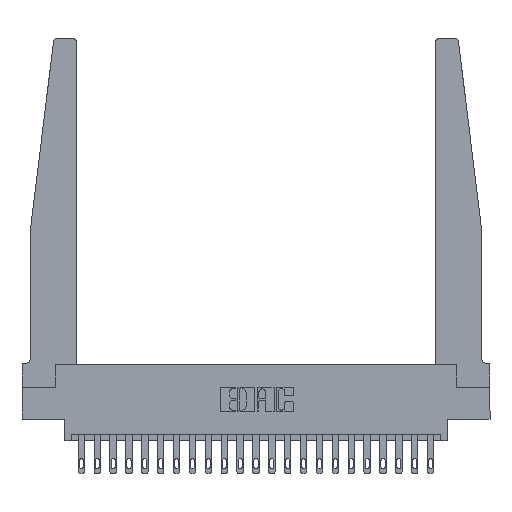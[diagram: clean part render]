
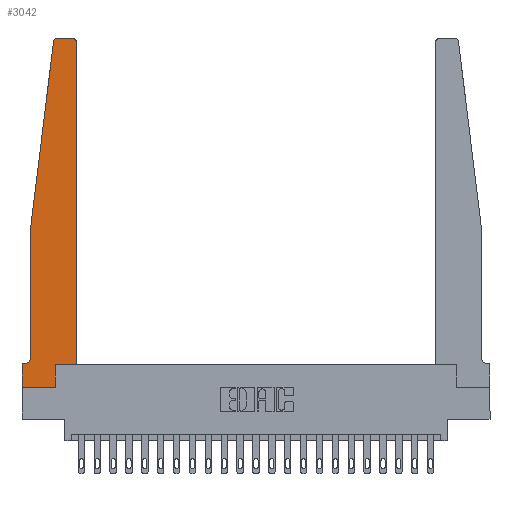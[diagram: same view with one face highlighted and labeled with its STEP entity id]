
A CAD part, top view. The second image highlights one B-rep face of the part: STEP entity #3042.
In plain terms, the highlighted planar face has unit normal (0, 0, 1).
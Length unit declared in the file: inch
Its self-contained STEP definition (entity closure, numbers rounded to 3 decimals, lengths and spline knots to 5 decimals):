
#126 = ORIENTED_EDGE ( 'NONE', *, *, #393, .T. ) ;
#183 = DIRECTION ( 'NONE',  ( 1., 0., 0. ) ) ;
#236 = EDGE_CURVE ( 'NONE', #21204, #19643, #19455, .T. ) ;
#339 = LINE ( 'NONE', #4034, #22434 ) ;
#393 = EDGE_CURVE ( 'NONE', #11549, #18079, #339, .T. ) ;
#488 = ORIENTED_EDGE ( 'NONE', *, *, #6149, .T. ) ;
#562 = LINE ( 'NONE', #2733, #3468 ) ;
#579 = CARTESIAN_POINT ( 'NONE',  ( 0.2605, 0., 0.37 ) ) ;
#1019 = VECTOR ( 'NONE', #183, 39.37008 ) ;
#1161 = CIRCLE ( 'NONE', #21125, 0.05 ) ;
#1341 = VERTEX_POINT ( 'NONE', #579 ) ;
#1373 = CARTESIAN_POINT ( 'NONE',  ( 0., 0., 0.37 ) ) ;
#1983 = DIRECTION ( 'NONE',  ( 0., 1., 0. ) ) ;
#2058 = ORIENTED_EDGE ( 'NONE', *, *, #16150, .T. ) ;
#2071 = EDGE_CURVE ( 'NONE', #16886, #1341, #15549, .T. ) ;
#2107 = VERTEX_POINT ( 'NONE', #3378 ) ;
#2175 = EDGE_CURVE ( 'NONE', #3802, #21111, #22815, .T. ) ;
#2733 = CARTESIAN_POINT ( 'NONE',  ( 0.065, 1.25, 0.37 ) ) ;
#2735 = CARTESIAN_POINT ( 'NONE',  ( 0.395, 2.75, 0.37 ) ) ;
#2737 = ORIENTED_EDGE ( 'NONE', *, *, #17236, .T. ) ;
#3042 = ADVANCED_FACE ( 'NONE', ( #12100 ), #17551, .T. ) ;
#3098 = LINE ( 'NONE', #1373, #10890 ) ;
#3378 = CARTESIAN_POINT ( 'NONE',  ( 0.065, 1.25, 0.37 ) ) ;
#3468 = VECTOR ( 'NONE', #5738, 39.37008 ) ;
#3543 = LINE ( 'NONE', #13959, #17802 ) ;
#3569 = CARTESIAN_POINT ( 'NONE',  ( 0.425, 0.18, 0.37 ) ) ;
#3802 = VERTEX_POINT ( 'NONE', #20123 ) ;
#3847 = VERTEX_POINT ( 'NONE', #2735 ) ;
#4034 = CARTESIAN_POINT ( 'NONE',  ( 0.065, 0.1875, 0.37 ) ) ;
#4398 = DIRECTION ( 'NONE',  ( 1., 0., 0. ) ) ;
#4827 = CARTESIAN_POINT ( 'NONE',  ( 0.2605, 0.18, 0.37 ) ) ;
#5040 = VECTOR ( 'NONE', #17931, 39.37008 ) ;
#5209 = CARTESIAN_POINT ( 'NONE',  ( 0.425, 0.18, 0.37 ) ) ;
#5293 = ORIENTED_EDGE ( 'NONE', *, *, #6008, .T. ) ;
#5613 = EDGE_CURVE ( 'NONE', #1341, #21204, #14254, .T. ) ;
#5738 = DIRECTION ( 'NONE',  ( -0.122, -0.992, 0. ) ) ;
#5776 = VERTEX_POINT ( 'NONE', #22312 ) ;
#6008 = EDGE_CURVE ( 'NONE', #11415, #11549, #1161, .T. ) ;
#6114 = AXIS2_PLACEMENT_3D ( 'NONE', #10316, #6827, #16087 ) ;
#6126 = ORIENTED_EDGE ( 'NONE', *, *, #2175, .T. ) ;
#6149 = EDGE_CURVE ( 'NONE', #2107, #11415, #3543, .T. ) ;
#6218 = CARTESIAN_POINT ( 'NONE',  ( 0.2605, 0.18, 0.37 ) ) ;
#6672 = DIRECTION ( 'NONE',  ( 0., 0., -1. ) ) ;
#6827 = DIRECTION ( 'NONE',  ( 0., 0., 1. ) ) ;
#8082 = CARTESIAN_POINT ( 'NONE',  ( 0.24675, 2.72367, 0.37 ) ) ;
#8585 = CARTESIAN_POINT ( 'NONE',  ( 0., 0., 0.37 ) ) ;
#8594 = DIRECTION ( 'NONE',  ( 0., 1., 0. ) ) ;
#8703 = CARTESIAN_POINT ( 'NONE',  ( 0., 0.1875, 0.37 ) ) ;
#8741 = DIRECTION ( 'NONE',  ( 0., -1., 0. ) ) ;
#8960 = DIRECTION ( 'NONE',  ( 0., 0., 1. ) ) ;
#9101 = AXIS2_PLACEMENT_3D ( 'NONE', #12213, #8960, #10258 ) ;
#9253 = CARTESIAN_POINT ( 'NONE',  ( 0.015, 0.1875, 0.37 ) ) ;
#10015 = VECTOR ( 'NONE', #1983, 39.37008 ) ;
#10258 = DIRECTION ( 'NONE',  ( 1., 0., 0. ) ) ;
#10316 = CARTESIAN_POINT ( 'NONE',  ( 0.395, 2.72, 0.37 ) ) ;
#10421 = DIRECTION ( 'NONE',  ( -1., 0., 0. ) ) ;
#10890 = VECTOR ( 'NONE', #17121, 39.37008 ) ;
#11081 = DIRECTION ( 'NONE',  ( -1., 0., 0. ) ) ;
#11367 = EDGE_CURVE ( 'NONE', #3847, #3802, #17147, .T. ) ;
#11415 = VERTEX_POINT ( 'NONE', #12507 ) ;
#11549 = VERTEX_POINT ( 'NONE', #9253 ) ;
#12100 = FACE_OUTER_BOUND ( 'NONE', #15609, .T. ) ;
#12213 = CARTESIAN_POINT ( 'NONE',  ( 0., 0.1875, 0.37 ) ) ;
#12330 = EDGE_CURVE ( 'NONE', #19643, #5776, #15768, .T. ) ;
#12507 = CARTESIAN_POINT ( 'NONE',  ( 0.065, 0.2375, 0.37 ) ) ;
#12791 = ORIENTED_EDGE ( 'NONE', *, *, #11367, .T. ) ;
#12871 = CARTESIAN_POINT ( 'NONE',  ( 0.27653, 2.72, 0.37 ) ) ;
#13204 = DIRECTION ( 'NONE',  ( 0., 0., 1. ) ) ;
#13959 = CARTESIAN_POINT ( 'NONE',  ( 0.065, 1.25, 0.37 ) ) ;
#14190 = ORIENTED_EDGE ( 'NONE', *, *, #2071, .T. ) ;
#14254 = LINE ( 'NONE', #6218, #10015 ) ;
#15469 = CARTESIAN_POINT ( 'NONE',  ( 0.015, 0.2375, 0.37 ) ) ;
#15549 = LINE ( 'NONE', #21343, #1019 ) ;
#15609 = EDGE_LOOP ( 'NONE', ( #12791, #6126, #2058, #488, #5293, #126, #2737, #14190, #16355, #22058, #17754, #21381 ) ) ;
#15768 = LINE ( 'NONE', #21114, #20055 ) ;
#16087 = DIRECTION ( 'NONE',  ( 1., 0., 0. ) ) ;
#16150 = EDGE_CURVE ( 'NONE', #21111, #2107, #562, .T. ) ;
#16355 = ORIENTED_EDGE ( 'NONE', *, *, #5613, .T. ) ;
#16886 = VERTEX_POINT ( 'NONE', #8585 ) ;
#17121 = DIRECTION ( 'NONE',  ( 0., -1., 0. ) ) ;
#17147 = LINE ( 'NONE', #17610, #20015 ) ;
#17236 = EDGE_CURVE ( 'NONE', #18079, #16886, #3098, .T. ) ;
#17551 = PLANE ( 'NONE',  #9101 ) ;
#17610 = CARTESIAN_POINT ( 'NONE',  ( 0.25, 2.75, 0.37 ) ) ;
#17656 = AXIS2_PLACEMENT_3D ( 'NONE', #12871, #13204, #4398 ) ;
#17754 = ORIENTED_EDGE ( 'NONE', *, *, #12330, .T. ) ;
#17802 = VECTOR ( 'NONE', #8741, 39.37008 ) ;
#17810 = DIRECTION ( 'NONE',  ( -1., 0., 0. ) ) ;
#17931 = DIRECTION ( 'NONE',  ( 1., 0., 0. ) ) ;
#18079 = VERTEX_POINT ( 'NONE', #8703 ) ;
#18636 = EDGE_CURVE ( 'NONE', #5776, #3847, #19822, .T. ) ;
#19455 = LINE ( 'NONE', #3569, #5040 ) ;
#19643 = VERTEX_POINT ( 'NONE', #5209 ) ;
#19822 = CIRCLE ( 'NONE', #6114, 0.03 ) ;
#20015 = VECTOR ( 'NONE', #10421, 39.37008 ) ;
#20055 = VECTOR ( 'NONE', #8594, 39.37008 ) ;
#20123 = CARTESIAN_POINT ( 'NONE',  ( 0.27653, 2.75, 0.37 ) ) ;
#21111 = VERTEX_POINT ( 'NONE', #8082 ) ;
#21114 = CARTESIAN_POINT ( 'NONE',  ( 0.425, 0.18, 0.37 ) ) ;
#21125 = AXIS2_PLACEMENT_3D ( 'NONE', #15469, #6672, #17810 ) ;
#21204 = VERTEX_POINT ( 'NONE', #4827 ) ;
#21343 = CARTESIAN_POINT ( 'NONE',  ( 0., 0., 0.37 ) ) ;
#21381 = ORIENTED_EDGE ( 'NONE', *, *, #18636, .T. ) ;
#22058 = ORIENTED_EDGE ( 'NONE', *, *, #236, .T. ) ;
#22312 = CARTESIAN_POINT ( 'NONE',  ( 0.425, 2.72, 0.37 ) ) ;
#22434 = VECTOR ( 'NONE', #11081, 39.37008 ) ;
#22815 = CIRCLE ( 'NONE', #17656, 0.03 ) ;
